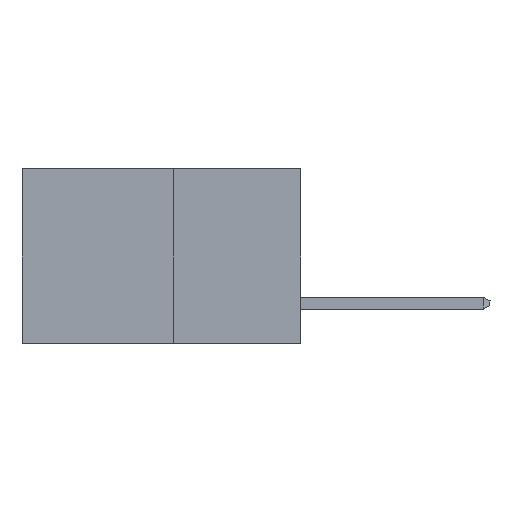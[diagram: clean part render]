
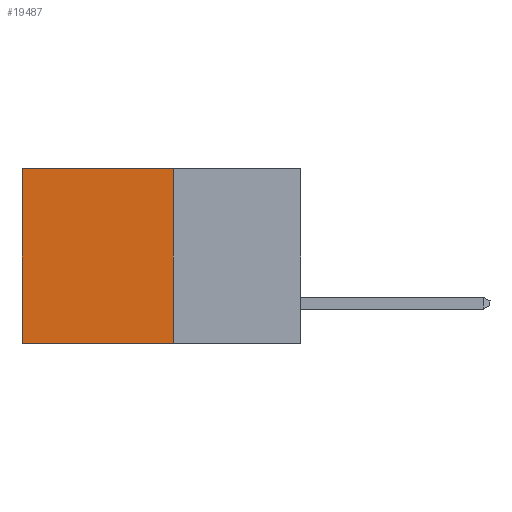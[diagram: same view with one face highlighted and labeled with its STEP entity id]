
A CAD part, left-side view. The second image highlights one B-rep face of the part: STEP entity #19487.
In plain terms, the highlighted planar face has unit normal (-1, 0, 0).
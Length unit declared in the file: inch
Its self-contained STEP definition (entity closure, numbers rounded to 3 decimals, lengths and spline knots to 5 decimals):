
#7 = VECTOR ( 'NONE', #13895, 39.37008 ) ;
#377 = VERTEX_POINT ( 'NONE', #18205 ) ;
#1310 = VERTEX_POINT ( 'NONE', #11805 ) ;
#1420 = CARTESIAN_POINT ( 'NONE',  ( 0.277, 0.59, 0. ) ) ;
#3322 = FACE_OUTER_BOUND ( 'NONE', #5836, .T. ) ;
#3553 = LINE ( 'NONE', #4581, #7276 ) ;
#4320 = VERTEX_POINT ( 'NONE', #1420 ) ;
#4498 = VECTOR ( 'NONE', #12186, 39.37008 ) ;
#4581 = CARTESIAN_POINT ( 'NONE',  ( 0.277, 0.27, -0.37 ) ) ;
#5280 = ORIENTED_EDGE ( 'NONE', *, *, #12218, .T. ) ;
#5836 = EDGE_LOOP ( 'NONE', ( #5280, #18226, #8305, #18987 ) ) ;
#6178 = DIRECTION ( 'NONE',  ( 0., 1., 0. ) ) ;
#7276 = VECTOR ( 'NONE', #6178, 39.37008 ) ;
#8305 = ORIENTED_EDGE ( 'NONE', *, *, #12910, .F. ) ;
#8581 = DIRECTION ( 'NONE',  ( 0., 0., -1. ) ) ;
#8886 = CARTESIAN_POINT ( 'NONE',  ( 0.277, 0.59, -0.37 ) ) ;
#9015 = CARTESIAN_POINT ( 'NONE',  ( 0.277, 0.59, -0.37 ) ) ;
#10683 = VECTOR ( 'NONE', #12489, 39.37008 ) ;
#10916 = CARTESIAN_POINT ( 'NONE',  ( 0.277, 0.27, 0. ) ) ;
#11805 = CARTESIAN_POINT ( 'NONE',  ( 0.277, 0.27, 0. ) ) ;
#12186 = DIRECTION ( 'NONE',  ( 0., 0., -1. ) ) ;
#12218 = EDGE_CURVE ( 'NONE', #4320, #20185, #17035, .T. ) ;
#12291 = CARTESIAN_POINT ( 'NONE',  ( 0.277, 0.27, -0.37 ) ) ;
#12489 = DIRECTION ( 'NONE',  ( 0., 1., 0. ) ) ;
#12910 = EDGE_CURVE ( 'NONE', #1310, #377, #16768, .T. ) ;
#13006 = EDGE_CURVE ( 'NONE', #1310, #4320, #18906, .T. ) ;
#13049 = AXIS2_PLACEMENT_3D ( 'NONE', #16372, #17880, #8581 ) ;
#13895 = DIRECTION ( 'NONE',  ( 0., 0., -1. ) ) ;
#16372 = CARTESIAN_POINT ( 'NONE',  ( 0.277, 0.27, -0.37 ) ) ;
#16768 = LINE ( 'NONE', #12291, #7 ) ;
#17035 = LINE ( 'NONE', #9015, #4498 ) ;
#17880 = DIRECTION ( 'NONE',  ( 1., 0., 0. ) ) ;
#18205 = CARTESIAN_POINT ( 'NONE',  ( 0.277, 0.27, -0.37 ) ) ;
#18226 = ORIENTED_EDGE ( 'NONE', *, *, #19690, .F. ) ;
#18906 = LINE ( 'NONE', #10916, #10683 ) ;
#18987 = ORIENTED_EDGE ( 'NONE', *, *, #13006, .T. ) ;
#19361 = PLANE ( 'NONE',  #13049 ) ;
#19487 = ADVANCED_FACE ( 'NONE', ( #3322 ), #19361, .F. ) ;
#19690 = EDGE_CURVE ( 'NONE', #377, #20185, #3553, .T. ) ;
#20185 = VERTEX_POINT ( 'NONE', #8886 ) ;
